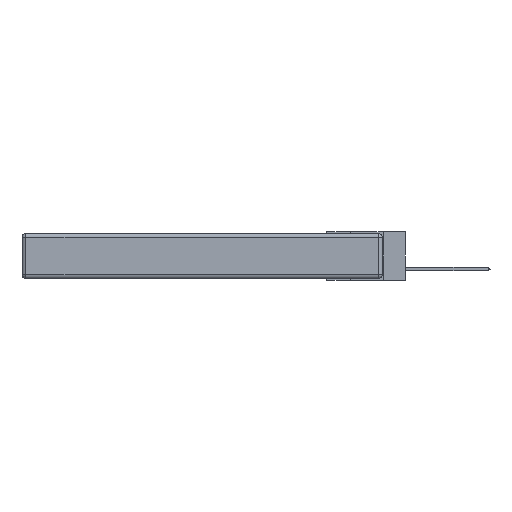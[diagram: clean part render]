
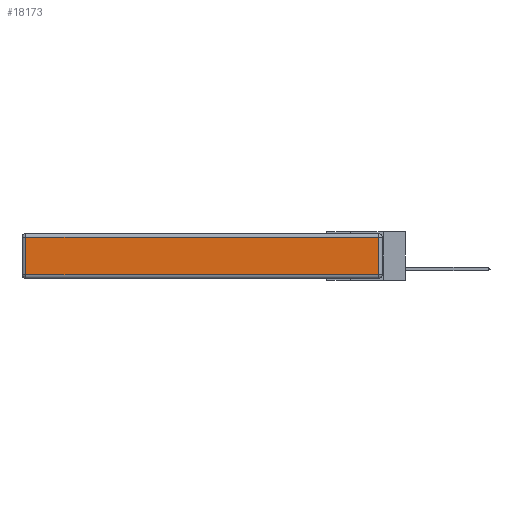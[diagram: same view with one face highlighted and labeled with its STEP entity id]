
A CAD part, left-side view. The second image highlights one B-rep face of the part: STEP entity #18173.
In plain terms, the highlighted planar face has unit normal (-1, 0, 0).
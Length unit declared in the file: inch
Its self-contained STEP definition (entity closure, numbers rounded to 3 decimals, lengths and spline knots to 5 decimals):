
#673 = VECTOR ( 'NONE', #12220, 39.37008 ) ;
#1232 = CARTESIAN_POINT ( 'NONE',  ( 0., 2.75, -0.03 ) ) ;
#1403 = DIRECTION ( 'NONE',  ( 0., 1., 0. ) ) ;
#2050 = CARTESIAN_POINT ( 'NONE',  ( 0., 2.72, -0.03 ) ) ;
#2189 = ORIENTED_EDGE ( 'NONE', *, *, #15826, .T. ) ;
#3673 = PLANE ( 'NONE',  #13382 ) ;
#4517 = CARTESIAN_POINT ( 'NONE',  ( 0., 0.03, -0.313 ) ) ;
#5619 = CARTESIAN_POINT ( 'NONE',  ( 0., 2.72, -0.343 ) ) ;
#6035 = LINE ( 'NONE', #5619, #673 ) ;
#6173 = VERTEX_POINT ( 'NONE', #24141 ) ;
#6257 = VECTOR ( 'NONE', #6598, 39.37008 ) ;
#6589 = EDGE_CURVE ( 'NONE', #15447, #15715, #25003, .T. ) ;
#6598 = DIRECTION ( 'NONE',  ( 0., 0., 1. ) ) ;
#6689 = EDGE_CURVE ( 'NONE', #15715, #6173, #6035, .T. ) ;
#9061 = EDGE_LOOP ( 'NONE', ( #12854, #2189, #15780, #13067 ) ) ;
#9816 = DIRECTION ( 'NONE',  ( 0., 0., 1. ) ) ;
#12220 = DIRECTION ( 'NONE',  ( 0., 0., -1. ) ) ;
#12634 = VECTOR ( 'NONE', #1403, 39.37008 ) ;
#12854 = ORIENTED_EDGE ( 'NONE', *, *, #21862, .T. ) ;
#13067 = ORIENTED_EDGE ( 'NONE', *, *, #6689, .T. ) ;
#13382 = AXIS2_PLACEMENT_3D ( 'NONE', #23798, #15558, #9816 ) ;
#13829 = CARTESIAN_POINT ( 'NONE',  ( 0., 0., -0.313 ) ) ;
#14553 = CARTESIAN_POINT ( 'NONE',  ( 0., 0.03, -0.343 ) ) ;
#15103 = FACE_OUTER_BOUND ( 'NONE', #9061, .T. ) ;
#15447 = VERTEX_POINT ( 'NONE', #15986 ) ;
#15558 = DIRECTION ( 'NONE',  ( -1., 0., 0. ) ) ;
#15715 = VERTEX_POINT ( 'NONE', #2050 ) ;
#15780 = ORIENTED_EDGE ( 'NONE', *, *, #6589, .T. ) ;
#15826 = EDGE_CURVE ( 'NONE', #24516, #15447, #19857, .T. ) ;
#15956 = DIRECTION ( 'NONE',  ( 0., -1., 0. ) ) ;
#15986 = CARTESIAN_POINT ( 'NONE',  ( 0., 0.03, -0.03 ) ) ;
#18173 = ADVANCED_FACE ( 'NONE', ( #15103 ), #3673, .T. ) ;
#19857 = LINE ( 'NONE', #14553, #6257 ) ;
#20902 = LINE ( 'NONE', #13829, #23782 ) ;
#21862 = EDGE_CURVE ( 'NONE', #6173, #24516, #20902, .T. ) ;
#23782 = VECTOR ( 'NONE', #15956, 39.37008 ) ;
#23798 = CARTESIAN_POINT ( 'NONE',  ( 0., 0., -0.343 ) ) ;
#24141 = CARTESIAN_POINT ( 'NONE',  ( 0., 2.72, -0.313 ) ) ;
#24516 = VERTEX_POINT ( 'NONE', #4517 ) ;
#25003 = LINE ( 'NONE', #1232, #12634 ) ;
